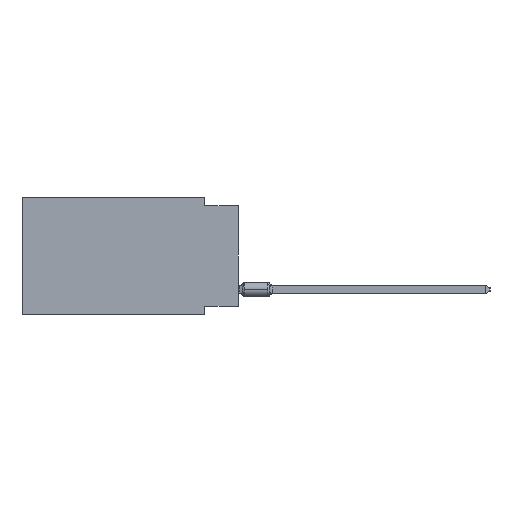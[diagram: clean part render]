
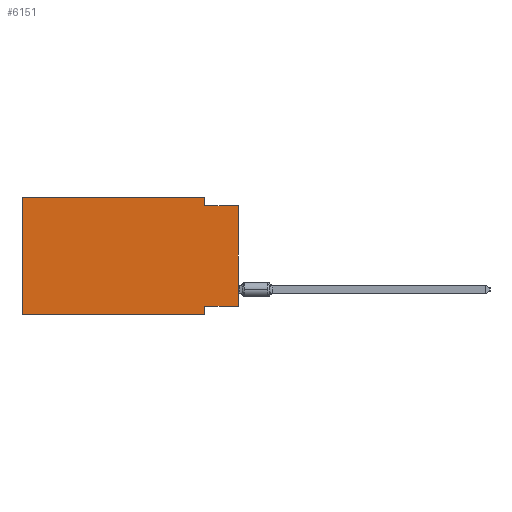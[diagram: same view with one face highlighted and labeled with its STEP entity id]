
A CAD part, left-side view. The second image highlights one B-rep face of the part: STEP entity #6151.
In plain terms, the highlighted planar face has unit normal (-1, 0, 0).
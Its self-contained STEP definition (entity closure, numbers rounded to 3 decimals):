
#48 = VECTOR ( 'NONE', #31220, 1000. ) ;
#1848 = ORIENTED_EDGE ( 'NONE', *, *, #5725, .F. ) ;
#1961 = LINE ( 'NONE', #21399, #39590 ) ;
#2324 = CARTESIAN_POINT ( 'NONE',  ( 0., 16.383, 0. ) ) ;
#2696 = EDGE_CURVE ( 'NONE', #21739, #4313, #12385, .T. ) ;
#4313 = VERTEX_POINT ( 'NONE', #39675 ) ;
#4437 = CARTESIAN_POINT ( 'NONE',  ( 0., 2.54, -8.89 ) ) ;
#4678 = VERTEX_POINT ( 'NONE', #6693 ) ;
#4718 = DIRECTION ( 'NONE',  ( 0., -1., 0. ) ) ;
#5604 = VECTOR ( 'NONE', #27215, 1000. ) ;
#5725 = EDGE_CURVE ( 'NONE', #35979, #9563, #37912, .T. ) ;
#6151 = ADVANCED_FACE ( 'NONE', ( #26984 ), #46916, .F. ) ;
#6693 = CARTESIAN_POINT ( 'NONE',  ( 0., 2.54, -8.89 ) ) ;
#7781 = CARTESIAN_POINT ( 'NONE',  ( 0., 16.383, 0. ) ) ;
#8068 = ORIENTED_EDGE ( 'NONE', *, *, #36840, .T. ) ;
#8543 = CARTESIAN_POINT ( 'NONE',  ( 0., 0., -0.635 ) ) ;
#8653 = EDGE_CURVE ( 'NONE', #16624, #4678, #19527, .T. ) ;
#9563 = VERTEX_POINT ( 'NONE', #10357 ) ;
#10095 = EDGE_LOOP ( 'NONE', ( #8068, #45371, #15624, #1848, #31065, #37026, #46235, #34336 ) ) ;
#10357 = CARTESIAN_POINT ( 'NONE',  ( 0., 2.54, 0. ) ) ;
#10823 = DIRECTION ( 'NONE',  ( 0., 0., 1. ) ) ;
#11517 = CARTESIAN_POINT ( 'NONE',  ( 0., 2.54, 0. ) ) ;
#12385 = LINE ( 'NONE', #8543, #24846 ) ;
#15448 = DIRECTION ( 'NONE',  ( 0., 1., 0. ) ) ;
#15614 = LINE ( 'NONE', #11517, #48 ) ;
#15624 = ORIENTED_EDGE ( 'NONE', *, *, #30577, .F. ) ;
#15742 = CARTESIAN_POINT ( 'NONE',  ( 0., 2.54, -0.635 ) ) ;
#16088 = VECTOR ( 'NONE', #30014, 1000. ) ;
#16624 = VERTEX_POINT ( 'NONE', #36802 ) ;
#18503 = CARTESIAN_POINT ( 'NONE',  ( 0., 0., -8.255 ) ) ;
#19527 = LINE ( 'NONE', #4437, #5604 ) ;
#21399 = CARTESIAN_POINT ( 'NONE',  ( 0., 16.383, 0. ) ) ;
#21739 = VERTEX_POINT ( 'NONE', #15742 ) ;
#21925 = EDGE_CURVE ( 'NONE', #23907, #4678, #35677, .T. ) ;
#22881 = DIRECTION ( 'NONE',  ( 0., 0., -1. ) ) ;
#23397 = CARTESIAN_POINT ( 'NONE',  ( 0., 16.383, -8.89 ) ) ;
#23907 = VERTEX_POINT ( 'NONE', #31828 ) ;
#24846 = VECTOR ( 'NONE', #4718, 1000. ) ;
#26696 = CARTESIAN_POINT ( 'NONE',  ( 0., 0., 0. ) ) ;
#26984 = FACE_OUTER_BOUND ( 'NONE', #10095, .T. ) ;
#27215 = DIRECTION ( 'NONE',  ( 0., 0., -1. ) ) ;
#27497 = DIRECTION ( 'NONE',  ( 1., 0., 0. ) ) ;
#27811 = VECTOR ( 'NONE', #10823, 1000. ) ;
#28354 = AXIS2_PLACEMENT_3D ( 'NONE', #7781, #27497, #22881 ) ;
#29598 = DIRECTION ( 'NONE',  ( 0., 0., 1. ) ) ;
#30014 = DIRECTION ( 'NONE',  ( 0., -1., 0. ) ) ;
#30577 = EDGE_CURVE ( 'NONE', #9563, #21739, #15614, .T. ) ;
#31065 = ORIENTED_EDGE ( 'NONE', *, *, #45631, .F. ) ;
#31220 = DIRECTION ( 'NONE',  ( 0., 0., -1. ) ) ;
#31339 = DIRECTION ( 'NONE',  ( 0., -1., 0. ) ) ;
#31828 = CARTESIAN_POINT ( 'NONE',  ( 0., 16.383, -8.89 ) ) ;
#33600 = VECTOR ( 'NONE', #31339, 1000. ) ;
#34336 = ORIENTED_EDGE ( 'NONE', *, *, #46159, .F. ) ;
#35677 = LINE ( 'NONE', #23397, #33600 ) ;
#35979 = VERTEX_POINT ( 'NONE', #2324 ) ;
#36802 = CARTESIAN_POINT ( 'NONE',  ( 0., 2.54, -8.255 ) ) ;
#36840 = EDGE_CURVE ( 'NONE', #36860, #4313, #46118, .T. ) ;
#36860 = VERTEX_POINT ( 'NONE', #18503 ) ;
#37026 = ORIENTED_EDGE ( 'NONE', *, *, #21925, .T. ) ;
#37912 = LINE ( 'NONE', #45084, #16088 ) ;
#38713 = CARTESIAN_POINT ( 'NONE',  ( 0., 0., -8.255 ) ) ;
#39590 = VECTOR ( 'NONE', #29598, 1000. ) ;
#39675 = CARTESIAN_POINT ( 'NONE',  ( 0., 0., -0.635 ) ) ;
#42555 = LINE ( 'NONE', #38713, #42887 ) ;
#42887 = VECTOR ( 'NONE', #15448, 1000. ) ;
#45084 = CARTESIAN_POINT ( 'NONE',  ( 0., 16.383, 0. ) ) ;
#45371 = ORIENTED_EDGE ( 'NONE', *, *, #2696, .F. ) ;
#45631 = EDGE_CURVE ( 'NONE', #23907, #35979, #1961, .T. ) ;
#46118 = LINE ( 'NONE', #26696, #27811 ) ;
#46159 = EDGE_CURVE ( 'NONE', #36860, #16624, #42555, .T. ) ;
#46235 = ORIENTED_EDGE ( 'NONE', *, *, #8653, .F. ) ;
#46916 = PLANE ( 'NONE',  #28354 ) ;
